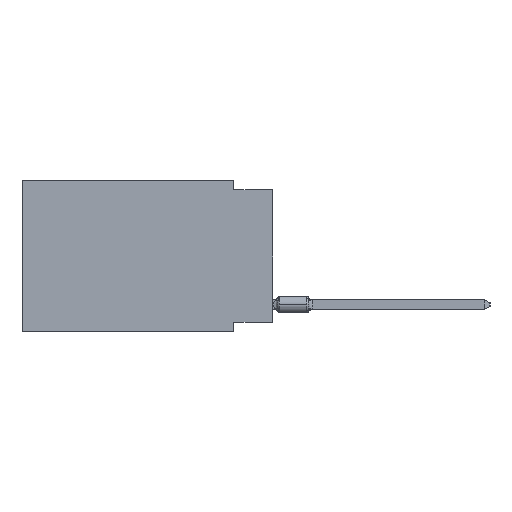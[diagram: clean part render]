
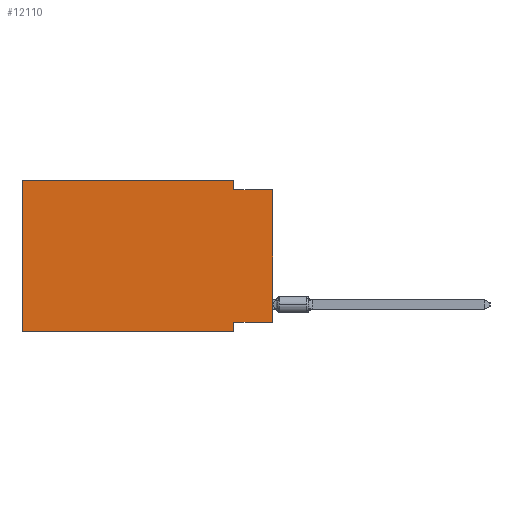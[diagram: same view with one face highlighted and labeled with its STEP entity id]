
A CAD part, left-side view. The second image highlights one B-rep face of the part: STEP entity #12110.
In plain terms, the highlighted planar face has unit normal (-1, 0, 0).
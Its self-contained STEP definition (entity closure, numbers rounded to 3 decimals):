
#1418 = DIRECTION ( 'NONE',  ( 0., 0., -1. ) ) ;
#2645 = LINE ( 'NONE', #10642, #38357 ) ;
#3660 = CARTESIAN_POINT ( 'NONE',  ( 0., 0., -9.271 ) ) ;
#4225 = CARTESIAN_POINT ( 'NONE',  ( 0., 2.54, 0. ) ) ;
#5294 = VECTOR ( 'NONE', #8267, 1000. ) ;
#5320 = ORIENTED_EDGE ( 'NONE', *, *, #43597, .F. ) ;
#5435 = VERTEX_POINT ( 'NONE', #4225 ) ;
#6126 = DIRECTION ( 'NONE',  ( 0., 0., -1. ) ) ;
#7146 = CARTESIAN_POINT ( 'NONE',  ( 0., 0., -0.635 ) ) ;
#8242 = CARTESIAN_POINT ( 'NONE',  ( 0., 2.54, -0.635 ) ) ;
#8267 = DIRECTION ( 'NONE',  ( 0., 1., 0. ) ) ;
#9114 = ORIENTED_EDGE ( 'NONE', *, *, #26707, .F. ) ;
#9955 = LINE ( 'NONE', #27040, #38133 ) ;
#10105 = VECTOR ( 'NONE', #45236, 1000. ) ;
#10490 = VERTEX_POINT ( 'NONE', #16917 ) ;
#10545 = AXIS2_PLACEMENT_3D ( 'NONE', #43221, #25426, #1418 ) ;
#10642 = CARTESIAN_POINT ( 'NONE',  ( 0., 16.383, 0. ) ) ;
#11392 = EDGE_LOOP ( 'NONE', ( #43870, #37985, #12415, #43542, #37276, #11394, #5320, #9114 ) ) ;
#11394 = ORIENTED_EDGE ( 'NONE', *, *, #20450, .T. ) ;
#11662 = VERTEX_POINT ( 'NONE', #15337 ) ;
#12110 = ADVANCED_FACE ( 'NONE', ( #28903 ), #14600, .F. ) ;
#12415 = ORIENTED_EDGE ( 'NONE', *, *, #41066, .F. ) ;
#13046 = EDGE_CURVE ( 'NONE', #14608, #10490, #37866, .T. ) ;
#13057 = LINE ( 'NONE', #16997, #36802 ) ;
#14016 = CARTESIAN_POINT ( 'NONE',  ( 0., 16.383, 0. ) ) ;
#14600 = PLANE ( 'NONE',  #10545 ) ;
#14608 = VERTEX_POINT ( 'NONE', #8242 ) ;
#14987 = LINE ( 'NONE', #18673, #35396 ) ;
#15337 = CARTESIAN_POINT ( 'NONE',  ( 0., 2.54, -9.271 ) ) ;
#16917 = CARTESIAN_POINT ( 'NONE',  ( 0., 0., -0.635 ) ) ;
#16997 = CARTESIAN_POINT ( 'NONE',  ( 0., 2.54, -9.906 ) ) ;
#18617 = CARTESIAN_POINT ( 'NONE',  ( 0., 16.383, 0. ) ) ;
#18673 = CARTESIAN_POINT ( 'NONE',  ( 0., 16.383, -9.906 ) ) ;
#19913 = EDGE_CURVE ( 'NONE', #35340, #5435, #2645, .T. ) ;
#20450 = EDGE_CURVE ( 'NONE', #22278, #31937, #14987, .T. ) ;
#21027 = VECTOR ( 'NONE', #42178, 1000. ) ;
#22278 = VERTEX_POINT ( 'NONE', #45092 ) ;
#22334 = CARTESIAN_POINT ( 'NONE',  ( 0., 0., -9.271 ) ) ;
#25426 = DIRECTION ( 'NONE',  ( 1., 0., 0. ) ) ;
#26032 = LINE ( 'NONE', #22334, #5294 ) ;
#26707 = EDGE_CURVE ( 'NONE', #33666, #11662, #26032, .T. ) ;
#27040 = CARTESIAN_POINT ( 'NONE',  ( 0., 0., 0. ) ) ;
#28141 = LINE ( 'NONE', #41537, #10105 ) ;
#28819 = CARTESIAN_POINT ( 'NONE',  ( 0., 2.54, -9.906 ) ) ;
#28903 = FACE_OUTER_BOUND ( 'NONE', #11392, .T. ) ;
#31937 = VERTEX_POINT ( 'NONE', #28819 ) ;
#33180 = EDGE_CURVE ( 'NONE', #33666, #10490, #9955, .T. ) ;
#33666 = VERTEX_POINT ( 'NONE', #3660 ) ;
#34501 = DIRECTION ( 'NONE',  ( 0., -1., 0. ) ) ;
#35311 = EDGE_CURVE ( 'NONE', #22278, #35340, #45653, .T. ) ;
#35340 = VERTEX_POINT ( 'NONE', #18617 ) ;
#35396 = VECTOR ( 'NONE', #35751, 1000. ) ;
#35751 = DIRECTION ( 'NONE',  ( 0., -1., 0. ) ) ;
#36802 = VECTOR ( 'NONE', #6126, 1000. ) ;
#37276 = ORIENTED_EDGE ( 'NONE', *, *, #35311, .F. ) ;
#37866 = LINE ( 'NONE', #7146, #40839 ) ;
#37985 = ORIENTED_EDGE ( 'NONE', *, *, #13046, .F. ) ;
#38133 = VECTOR ( 'NONE', #41815, 1000. ) ;
#38357 = VECTOR ( 'NONE', #34501, 1000. ) ;
#40839 = VECTOR ( 'NONE', #45044, 1000. ) ;
#41066 = EDGE_CURVE ( 'NONE', #5435, #14608, #28141, .T. ) ;
#41537 = CARTESIAN_POINT ( 'NONE',  ( 0., 2.54, 0. ) ) ;
#41815 = DIRECTION ( 'NONE',  ( 0., 0., 1. ) ) ;
#42178 = DIRECTION ( 'NONE',  ( 0., 0., 1. ) ) ;
#43221 = CARTESIAN_POINT ( 'NONE',  ( 0., 16.383, 0. ) ) ;
#43542 = ORIENTED_EDGE ( 'NONE', *, *, #19913, .F. ) ;
#43597 = EDGE_CURVE ( 'NONE', #11662, #31937, #13057, .T. ) ;
#43870 = ORIENTED_EDGE ( 'NONE', *, *, #33180, .T. ) ;
#45044 = DIRECTION ( 'NONE',  ( 0., -1., 0. ) ) ;
#45092 = CARTESIAN_POINT ( 'NONE',  ( 0., 16.383, -9.906 ) ) ;
#45236 = DIRECTION ( 'NONE',  ( 0., 0., -1. ) ) ;
#45653 = LINE ( 'NONE', #14016, #21027 ) ;
